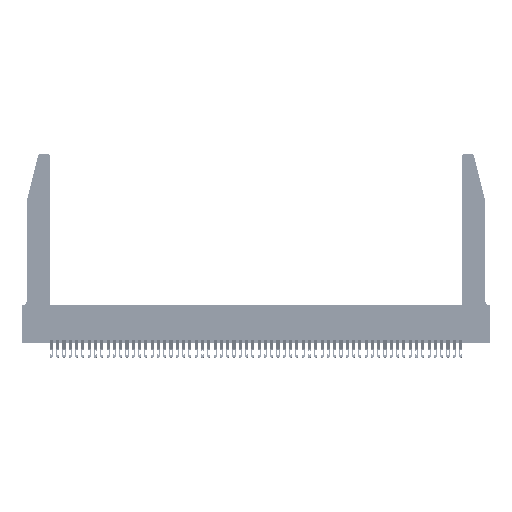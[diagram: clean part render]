
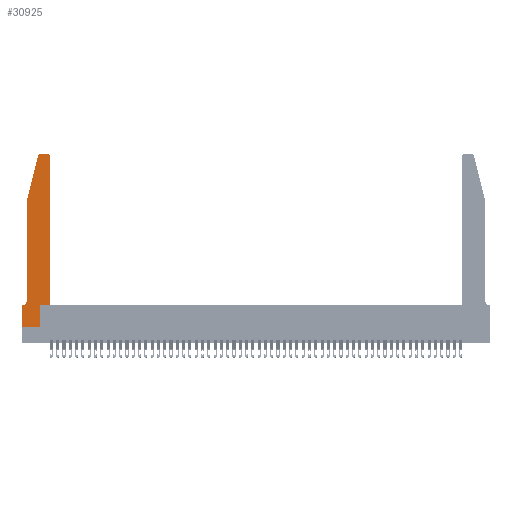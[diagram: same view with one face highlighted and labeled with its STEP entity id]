
A CAD part, top view. The second image highlights one B-rep face of the part: STEP entity #30925.
In plain terms, the highlighted planar face has unit normal (0, 0, 1).
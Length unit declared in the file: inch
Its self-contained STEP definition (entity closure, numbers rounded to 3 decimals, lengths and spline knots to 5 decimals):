
#171 = VECTOR ( 'NONE', #47753, 39.37008 ) ;
#937 = DIRECTION ( 'NONE',  ( -0.239, -0.971, 0. ) ) ;
#1103 = LINE ( 'NONE', #30605, #53594 ) ;
#1404 = ORIENTED_EDGE ( 'NONE', *, *, #19033, .T. ) ;
#1493 = LINE ( 'NONE', #18974, #171 ) ;
#1788 = EDGE_CURVE ( 'NONE', #7815, #5312, #1944, .T. ) ;
#1806 = CARTESIAN_POINT ( 'NONE',  ( 0.284, 2.75, 0.37 ) ) ;
#1876 = DIRECTION ( 'NONE',  ( 0., 0., 1. ) ) ;
#1884 = VERTEX_POINT ( 'NONE', #21053 ) ;
#1944 = LINE ( 'NONE', #36571, #21624 ) ;
#2486 = VERTEX_POINT ( 'NONE', #16757 ) ;
#3546 = DIRECTION ( 'NONE',  ( 0., 0., -1. ) ) ;
#4371 = CIRCLE ( 'NONE', #39817, 0.03 ) ;
#4406 = CARTESIAN_POINT ( 'NONE',  ( 0., 0.35, 0.37 ) ) ;
#4867 = VECTOR ( 'NONE', #51347, 39.37008 ) ;
#4976 = DIRECTION ( 'NONE',  ( -1., 0., 0. ) ) ;
#5312 = VERTEX_POINT ( 'NONE', #1806 ) ;
#5383 = VECTOR ( 'NONE', #53501, 39.37008 ) ;
#5589 = LINE ( 'NONE', #38265, #14110 ) ;
#6959 = CARTESIAN_POINT ( 'NONE',  ( 0.4205, 2.72, 0.37 ) ) ;
#7076 = CARTESIAN_POINT ( 'NONE',  ( 0.4505, 0.35, 0.37 ) ) ;
#7634 = VECTOR ( 'NONE', #13274, 39.37008 ) ;
#7815 = VERTEX_POINT ( 'NONE', #13458 ) ;
#8392 = CARTESIAN_POINT ( 'NONE',  ( 0.0055, 0.35, 0.37 ) ) ;
#10048 = EDGE_CURVE ( 'NONE', #5312, #43380, #4371, .T. ) ;
#10984 = ORIENTED_EDGE ( 'NONE', *, *, #33792, .T. ) ;
#11153 = DIRECTION ( 'NONE',  ( 1., 0., 0. ) ) ;
#11440 = VERTEX_POINT ( 'NONE', #24486 ) ;
#12177 = VECTOR ( 'NONE', #22044, 39.37008 ) ;
#13274 = DIRECTION ( 'NONE',  ( 0., -1., 0. ) ) ;
#13424 = CIRCLE ( 'NONE', #33793, 0.03 ) ;
#13458 = CARTESIAN_POINT ( 'NONE',  ( 0.4205, 2.75, 0.37 ) ) ;
#14110 = VECTOR ( 'NONE', #4976, 39.37008 ) ;
#14776 = AXIS2_PLACEMENT_3D ( 'NONE', #4406, #21322, #50048 ) ;
#16757 = CARTESIAN_POINT ( 'NONE',  ( 0.0755, 2., 0.37 ) ) ;
#17493 = LINE ( 'NONE', #46195, #7634 ) ;
#17807 = CARTESIAN_POINT ( 'NONE',  ( 0.0755, 2., 0.37 ) ) ;
#18034 = ORIENTED_EDGE ( 'NONE', *, *, #37321, .T. ) ;
#18329 = ORIENTED_EDGE ( 'NONE', *, *, #32464, .T. ) ;
#18974 = CARTESIAN_POINT ( 'NONE',  ( 0.2865, 0.35, 0.37 ) ) ;
#19033 = EDGE_CURVE ( 'NONE', #11440, #32827, #49373, .T. ) ;
#19289 = VECTOR ( 'NONE', #937, 39.37008 ) ;
#21033 = CARTESIAN_POINT ( 'NONE',  ( 0.2865, 0., 0.37 ) ) ;
#21053 = CARTESIAN_POINT ( 'NONE',  ( 0.4505, 2.72, 0.37 ) ) ;
#21322 = DIRECTION ( 'NONE',  ( 0., 0., 1. ) ) ;
#21624 = VECTOR ( 'NONE', #44616, 39.37008 ) ;
#22044 = DIRECTION ( 'NONE',  ( 1., 0., 0. ) ) ;
#22251 = ORIENTED_EDGE ( 'NONE', *, *, #31048, .T. ) ;
#23255 = ORIENTED_EDGE ( 'NONE', *, *, #1788, .T. ) ;
#24486 = CARTESIAN_POINT ( 'NONE',  ( 0.0755, 0.42, 0.37 ) ) ;
#24575 = CARTESIAN_POINT ( 'NONE',  ( 0., 0., 0.37 ) ) ;
#25218 = AXIS2_PLACEMENT_3D ( 'NONE', #28584, #3546, #32700 ) ;
#26929 = CARTESIAN_POINT ( 'NONE',  ( 0.284, 2.72, 0.37 ) ) ;
#28584 = CARTESIAN_POINT ( 'NONE',  ( 0.0055, 0.42, 0.37 ) ) ;
#29726 = LINE ( 'NONE', #47213, #4867 ) ;
#30244 = LINE ( 'NONE', #41122, #5383 ) ;
#30605 = CARTESIAN_POINT ( 'NONE',  ( 0.4505, 0.35, 0.37 ) ) ;
#30925 = ADVANCED_FACE ( 'NONE', ( #51635 ), #33568, .T. ) ;
#31048 = EDGE_CURVE ( 'NONE', #32939, #50903, #46483, .T. ) ;
#31082 = DIRECTION ( 'NONE',  ( 1., 0., 0. ) ) ;
#31863 = EDGE_CURVE ( 'NONE', #47084, #37101, #29726, .T. ) ;
#32069 = VERTEX_POINT ( 'NONE', #52416 ) ;
#32134 = ORIENTED_EDGE ( 'NONE', *, *, #51139, .T. ) ;
#32464 = EDGE_CURVE ( 'NONE', #43380, #2486, #41213, .T. ) ;
#32700 = DIRECTION ( 'NONE',  ( -1., 0., 0. ) ) ;
#32827 = VERTEX_POINT ( 'NONE', #8392 ) ;
#32939 = VERTEX_POINT ( 'NONE', #42108 ) ;
#33568 = PLANE ( 'NONE',  #14776 ) ;
#33792 = EDGE_CURVE ( 'NONE', #37101, #32939, #1493, .T. ) ;
#33793 = AXIS2_PLACEMENT_3D ( 'NONE', #6959, #36075, #11153 ) ;
#34770 = ORIENTED_EDGE ( 'NONE', *, *, #10048, .T. ) ;
#36075 = DIRECTION ( 'NONE',  ( 0., 0., 1. ) ) ;
#36571 = CARTESIAN_POINT ( 'NONE',  ( 0.2605, 2.75, 0.37 ) ) ;
#37101 = VERTEX_POINT ( 'NONE', #21033 ) ;
#37321 = EDGE_CURVE ( 'NONE', #50903, #1884, #1103, .T. ) ;
#37937 = EDGE_CURVE ( 'NONE', #32827, #32069, #5589, .T. ) ;
#38190 = EDGE_CURVE ( 'NONE', #1884, #7815, #13424, .T. ) ;
#38265 = CARTESIAN_POINT ( 'NONE',  ( 0.0755, 0.35, 0.37 ) ) ;
#39661 = EDGE_CURVE ( 'NONE', #2486, #11440, #30244, .T. ) ;
#39817 = AXIS2_PLACEMENT_3D ( 'NONE', #26929, #1876, #31082 ) ;
#41122 = CARTESIAN_POINT ( 'NONE',  ( 0.0755, 2., 0.37 ) ) ;
#41213 = LINE ( 'NONE', #17807, #19289 ) ;
#42108 = CARTESIAN_POINT ( 'NONE',  ( 0.2865, 0.35, 0.37 ) ) ;
#42527 = CARTESIAN_POINT ( 'NONE',  ( 0.4505, 0.35, 0.37 ) ) ;
#43380 = VERTEX_POINT ( 'NONE', #47934 ) ;
#44616 = DIRECTION ( 'NONE',  ( -1., 0., 0. ) ) ;
#46195 = CARTESIAN_POINT ( 'NONE',  ( 0., 0., 0.37 ) ) ;
#46356 = ORIENTED_EDGE ( 'NONE', *, *, #37937, .T. ) ;
#46483 = LINE ( 'NONE', #42527, #12177 ) ;
#46676 = ORIENTED_EDGE ( 'NONE', *, *, #39661, .T. ) ;
#47070 = DIRECTION ( 'NONE',  ( 0., 1., 0. ) ) ;
#47084 = VERTEX_POINT ( 'NONE', #24575 ) ;
#47213 = CARTESIAN_POINT ( 'NONE',  ( 0., 0., 0.37 ) ) ;
#47527 = ORIENTED_EDGE ( 'NONE', *, *, #31863, .T. ) ;
#47753 = DIRECTION ( 'NONE',  ( 0., 1., 0. ) ) ;
#47934 = CARTESIAN_POINT ( 'NONE',  ( 0.25487, 2.72718, 0.37 ) ) ;
#49373 = CIRCLE ( 'NONE', #25218, 0.07 ) ;
#50041 = EDGE_LOOP ( 'NONE', ( #23255, #34770, #18329, #46676, #1404, #46356, #32134, #47527, #10984, #22251, #18034, #52631 ) ) ;
#50048 = DIRECTION ( 'NONE',  ( 1., 0., 0. ) ) ;
#50903 = VERTEX_POINT ( 'NONE', #7076 ) ;
#51139 = EDGE_CURVE ( 'NONE', #32069, #47084, #17493, .T. ) ;
#51347 = DIRECTION ( 'NONE',  ( 1., 0., 0. ) ) ;
#51635 = FACE_OUTER_BOUND ( 'NONE', #50041, .T. ) ;
#52416 = CARTESIAN_POINT ( 'NONE',  ( 0., 0.35, 0.37 ) ) ;
#52631 = ORIENTED_EDGE ( 'NONE', *, *, #38190, .T. ) ;
#53501 = DIRECTION ( 'NONE',  ( 0., -1., 0. ) ) ;
#53594 = VECTOR ( 'NONE', #47070, 39.37008 ) ;
